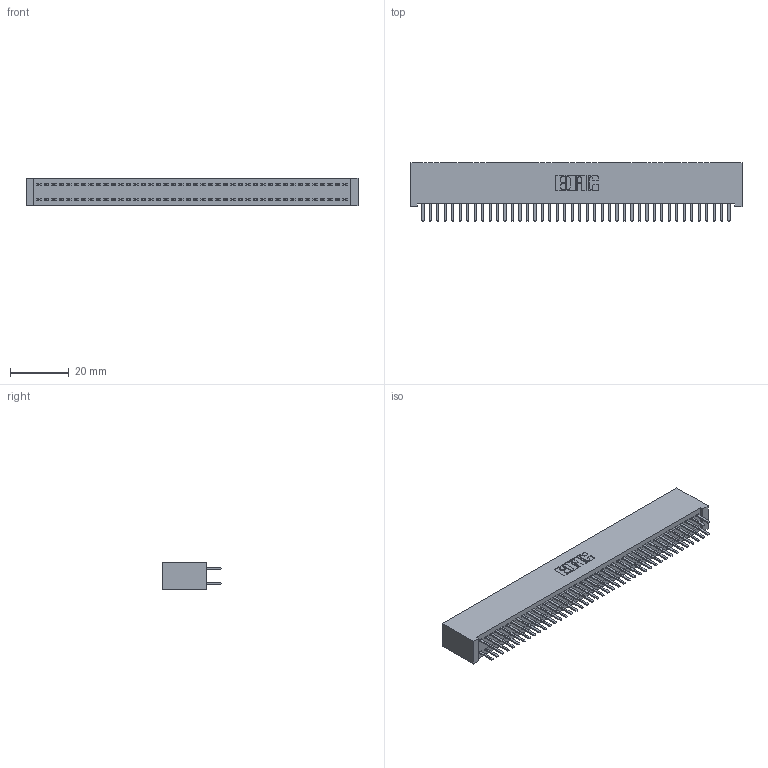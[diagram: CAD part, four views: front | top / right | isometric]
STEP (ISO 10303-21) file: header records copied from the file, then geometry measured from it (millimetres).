
FILE_DESCRIPTION (( 'STEP AP203' ), '1' );
FILE_NAME ('392-084-520-201.STEP', '2019-10-09T15:25:05', ( '' ), ( '' ), 'SwSTEP 2.0', 'SolidWorks 2016', '' );
FILE_SCHEMA (( 'CONFIG_CONTROL_DESIGN' ));
Length unit declared in the file: inch
Products named in the file (3): 342 Part_Lugless; 345-292-001_345-293-120; 392-084-520-201
Assembly tree (85 placements, depth 2):
  392-084-520-201
    342 Part_Lugless
    345-292-001_345-293-120  x84
Bounding box: 112.93 x 20.02 x 9.4 mm (x, y, z)
Volume: 10549.2 mm3; surface area: 17530.5 mm2
Topology: 85 solids, 85 shells, 4806 faces, 13967 edges, 9086 vertices
Faces by surface type: plane 3254, cylinder 1552
Entity records: 26725 total; most frequent: CARTESIAN_POINT 4438, ORIENTED_EDGE 4362, DIRECTION 3773, EDGE_CURVE 2181, VECTOR 2057, LINE 2057, VERTEX_POINT 1450, AXIS2_PLACEMENT_3D 858
